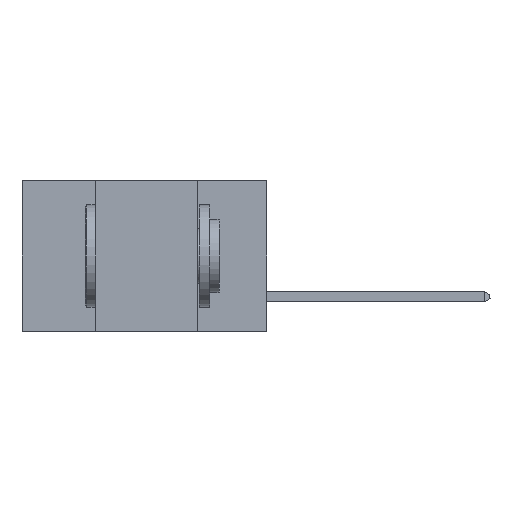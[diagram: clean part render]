
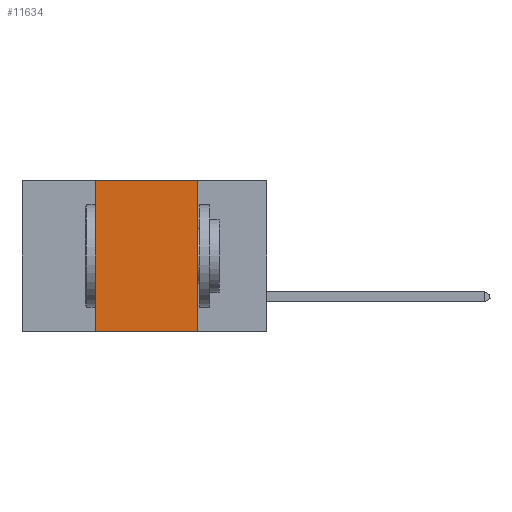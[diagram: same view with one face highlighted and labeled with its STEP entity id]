
A CAD part, left-side view. The second image highlights one B-rep face of the part: STEP entity #11634.
In plain terms, the highlighted planar face has unit normal (-1, 0, 0).
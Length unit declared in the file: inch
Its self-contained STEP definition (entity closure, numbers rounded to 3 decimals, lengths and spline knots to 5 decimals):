
#54 = CARTESIAN_POINT ( 'NONE',  ( 0., 0.17, 0. ) ) ;
#90 = ORIENTED_EDGE ( 'NONE', *, *, #3303, .F. ) ;
#554 = VERTEX_POINT ( 'NONE', #5254 ) ;
#598 = CARTESIAN_POINT ( 'NONE',  ( 0., 0.42, 0. ) ) ;
#1822 = CARTESIAN_POINT ( 'NONE',  ( 0., 0.6, 0. ) ) ;
#2253 = CARTESIAN_POINT ( 'NONE',  ( 0., 0.17, 0. ) ) ;
#2469 = VECTOR ( 'NONE', #11511, 39.37008 ) ;
#3066 = DIRECTION ( 'NONE',  ( 0., -1., 0. ) ) ;
#3303 = EDGE_CURVE ( 'NONE', #11129, #11739, #11508, .T. ) ;
#3818 = EDGE_CURVE ( 'NONE', #554, #4720, #8299, .T. ) ;
#4430 = EDGE_CURVE ( 'NONE', #554, #11129, #10616, .T. ) ;
#4588 = CARTESIAN_POINT ( 'NONE',  ( 0., 0.6, 0. ) ) ;
#4704 = VECTOR ( 'NONE', #7422, 39.37008 ) ;
#4720 = VERTEX_POINT ( 'NONE', #4725 ) ;
#4725 = CARTESIAN_POINT ( 'NONE',  ( 0., 0.17, -0.37 ) ) ;
#5167 = EDGE_LOOP ( 'NONE', ( #11457, #90, #6696, #9980 ) ) ;
#5254 = CARTESIAN_POINT ( 'NONE',  ( 0., 0.42, -0.37 ) ) ;
#5434 = FACE_OUTER_BOUND ( 'NONE', #5167, .T. ) ;
#5495 = DIRECTION ( 'NONE',  ( 1., 0., 0. ) ) ;
#5982 = VECTOR ( 'NONE', #3066, 39.37008 ) ;
#6421 = AXIS2_PLACEMENT_3D ( 'NONE', #4588, #5495, #9154 ) ;
#6696 = ORIENTED_EDGE ( 'NONE', *, *, #4430, .F. ) ;
#6929 = DIRECTION ( 'NONE',  ( 0., 0., 1. ) ) ;
#7422 = DIRECTION ( 'NONE',  ( 0., -1., 0. ) ) ;
#7547 = CARTESIAN_POINT ( 'NONE',  ( 0., 0.6, -0.37 ) ) ;
#7568 = VECTOR ( 'NONE', #6929, 39.37008 ) ;
#8299 = LINE ( 'NONE', #7547, #5982 ) ;
#9154 = DIRECTION ( 'NONE',  ( 0., 0., -1. ) ) ;
#9465 = EDGE_CURVE ( 'NONE', #11739, #4720, #11577, .T. ) ;
#9980 = ORIENTED_EDGE ( 'NONE', *, *, #3818, .T. ) ;
#10616 = LINE ( 'NONE', #11614, #7568 ) ;
#11129 = VERTEX_POINT ( 'NONE', #598 ) ;
#11457 = ORIENTED_EDGE ( 'NONE', *, *, #9465, .F. ) ;
#11508 = LINE ( 'NONE', #1822, #4704 ) ;
#11511 = DIRECTION ( 'NONE',  ( 0., 0., -1. ) ) ;
#11577 = LINE ( 'NONE', #2253, #2469 ) ;
#11614 = CARTESIAN_POINT ( 'NONE',  ( 0., 0.42, 0. ) ) ;
#11634 = ADVANCED_FACE ( 'NONE', ( #5434 ), #11956, .F. ) ;
#11739 = VERTEX_POINT ( 'NONE', #54 ) ;
#11956 = PLANE ( 'NONE',  #6421 ) ;
